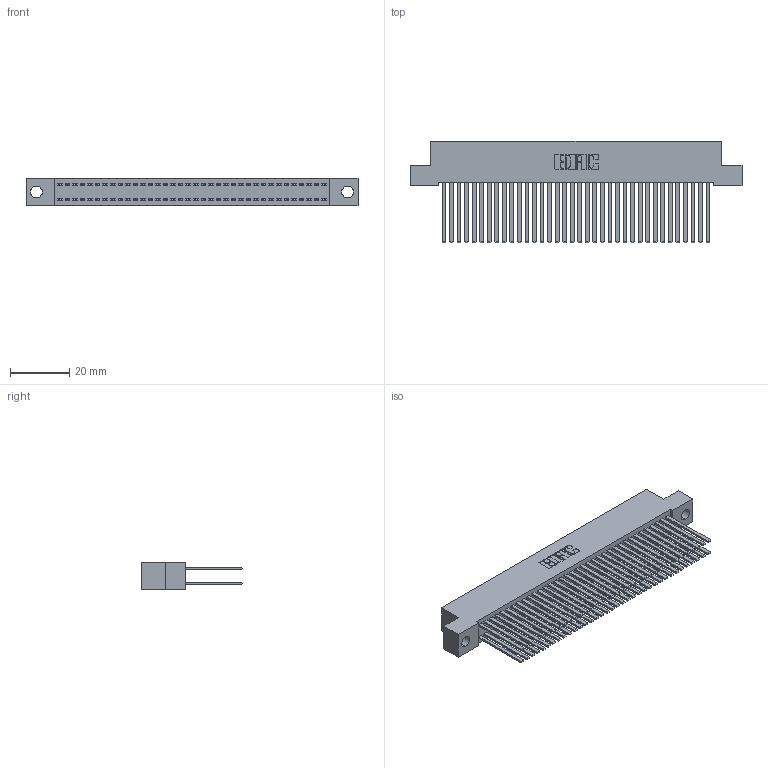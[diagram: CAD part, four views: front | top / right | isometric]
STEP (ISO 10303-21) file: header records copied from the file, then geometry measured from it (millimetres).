
FILE_DESCRIPTION (( 'STEP AP203' ), '1' );
FILE_NAME ('392-072-544-204.STEP', '2019-10-09T12:37:34', ( '' ), ( '' ), 'SwSTEP 2.0', 'SolidWorks 2016', '' );
FILE_SCHEMA (( 'CONFIG_CONTROL_DESIGN' ));
Length unit declared in the file: inch
Products named in the file (3): 345-292-001_345-293-144; 342 Part_.156 TH; 392-072-544-204
Assembly tree (73 placements, depth 2):
  392-072-544-204
    342 Part_.156 TH
    345-292-001_345-293-144  x72
Bounding box: 111.76 x 34.3 x 9.4 mm (x, y, z)
Volume: 10935.5 mm3; surface area: 20271.7 mm2
Topology: 73 solids, 73 shells, 3422 faces, 10163 edges, 6678 vertices
Faces by surface type: plane 2370, cylinder 1052
Entity records: 23623 total; most frequent: CARTESIAN_POINT 3918, ORIENTED_EDGE 3854, DIRECTION 3355, EDGE_CURVE 1927, VECTOR 1803, LINE 1803, VERTEX_POINT 1282, AXIS2_PLACEMENT_3D 776
